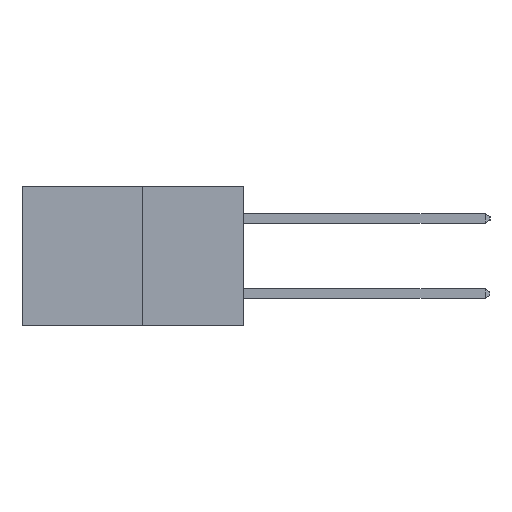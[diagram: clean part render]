
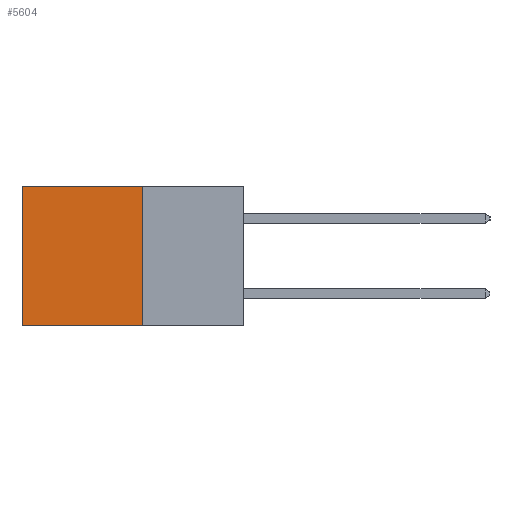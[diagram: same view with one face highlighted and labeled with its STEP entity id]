
A CAD part, left-side view. The second image highlights one B-rep face of the part: STEP entity #5604.
In plain terms, the highlighted planar face has unit normal (-1, 0, 0).
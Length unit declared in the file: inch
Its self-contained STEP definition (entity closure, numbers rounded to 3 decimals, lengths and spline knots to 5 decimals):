
#90 = CARTESIAN_POINT ( 'NONE',  ( 0.277, 0.59, 0. ) ) ;
#263 = VERTEX_POINT ( 'NONE', #3314 ) ;
#540 = VERTEX_POINT ( 'NONE', #5684 ) ;
#1025 = CARTESIAN_POINT ( 'NONE',  ( 0.277, 0.27, -0.37 ) ) ;
#1106 = ORIENTED_EDGE ( 'NONE', *, *, #7407, .F. ) ;
#1599 = VECTOR ( 'NONE', #12020, 39.37008 ) ;
#1785 = EDGE_CURVE ( 'NONE', #263, #9074, #3517, .T. ) ;
#2772 = CARTESIAN_POINT ( 'NONE',  ( 0.277, 0.27, 0. ) ) ;
#3314 = CARTESIAN_POINT ( 'NONE',  ( 0.277, 0.27, 0. ) ) ;
#3517 = LINE ( 'NONE', #2772, #6468 ) ;
#3761 = VERTEX_POINT ( 'NONE', #7963 ) ;
#3790 = DIRECTION ( 'NONE',  ( 0., 0., -1. ) ) ;
#4706 = ORIENTED_EDGE ( 'NONE', *, *, #12509, .F. ) ;
#4789 = DIRECTION ( 'NONE',  ( 0., 1., 0. ) ) ;
#4977 = AXIS2_PLACEMENT_3D ( 'NONE', #9248, #8097, #3790 ) ;
#5086 = CARTESIAN_POINT ( 'NONE',  ( 0.277, 0.27, -0.37 ) ) ;
#5388 = FACE_OUTER_BOUND ( 'NONE', #12639, .T. ) ;
#5604 = ADVANCED_FACE ( 'NONE', ( #5388 ), #8125, .F. ) ;
#5684 = CARTESIAN_POINT ( 'NONE',  ( 0.277, 0.27, -0.37 ) ) ;
#6468 = VECTOR ( 'NONE', #12086, 39.37008 ) ;
#7407 = EDGE_CURVE ( 'NONE', #540, #3761, #11443, .T. ) ;
#7434 = LINE ( 'NONE', #5086, #13166 ) ;
#7963 = CARTESIAN_POINT ( 'NONE',  ( 0.277, 0.59, -0.37 ) ) ;
#7965 = EDGE_CURVE ( 'NONE', #9074, #3761, #10048, .T. ) ;
#8097 = DIRECTION ( 'NONE',  ( 1., 0., 0. ) ) ;
#8125 = PLANE ( 'NONE',  #4977 ) ;
#8552 = VECTOR ( 'NONE', #4789, 39.37008 ) ;
#8717 = CARTESIAN_POINT ( 'NONE',  ( 0.277, 0.59, -0.37 ) ) ;
#9074 = VERTEX_POINT ( 'NONE', #90 ) ;
#9248 = CARTESIAN_POINT ( 'NONE',  ( 0.277, 0.27, -0.37 ) ) ;
#10048 = LINE ( 'NONE', #8717, #1599 ) ;
#10557 = ORIENTED_EDGE ( 'NONE', *, *, #1785, .T. ) ;
#11222 = ORIENTED_EDGE ( 'NONE', *, *, #7965, .T. ) ;
#11443 = LINE ( 'NONE', #1025, #8552 ) ;
#12020 = DIRECTION ( 'NONE',  ( 0., 0., -1. ) ) ;
#12086 = DIRECTION ( 'NONE',  ( 0., 1., 0. ) ) ;
#12509 = EDGE_CURVE ( 'NONE', #263, #540, #7434, .T. ) ;
#12639 = EDGE_LOOP ( 'NONE', ( #11222, #1106, #4706, #10557 ) ) ;
#12665 = DIRECTION ( 'NONE',  ( 0., 0., -1. ) ) ;
#13166 = VECTOR ( 'NONE', #12665, 39.37008 ) ;
